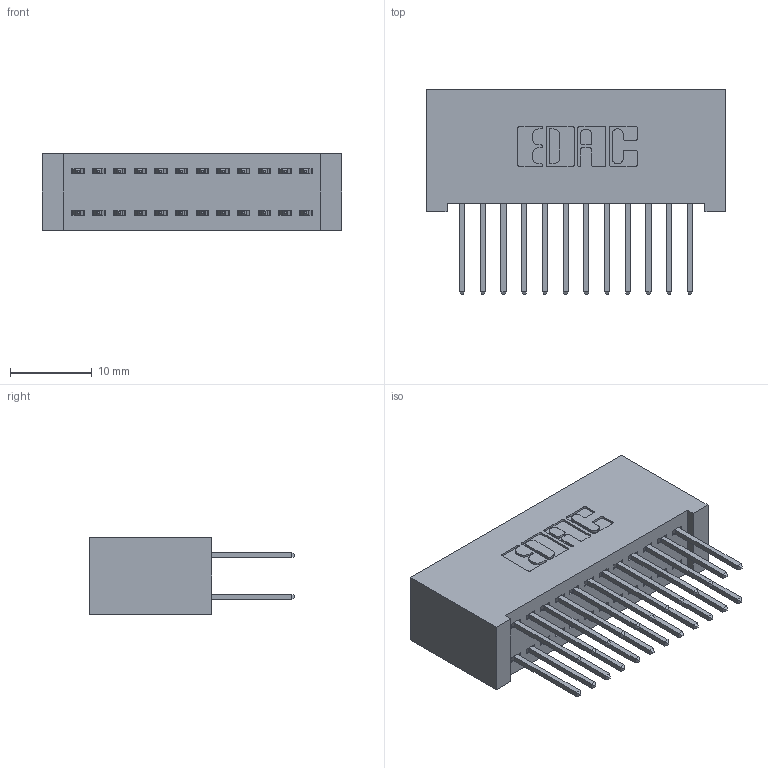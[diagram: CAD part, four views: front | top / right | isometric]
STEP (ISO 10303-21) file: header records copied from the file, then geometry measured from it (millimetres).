
FILE_DESCRIPTION (( 'STEP AP203' ), '1' );
FILE_NAME ('342-024-523-201.STEP', '2018-08-11T02:12:16', ( '' ), ( '' ), 'SwSTEP 2.0', 'SolidWorks 2016', '' );
FILE_SCHEMA (( 'CONFIG_CONTROL_DESIGN' ));
Length unit declared in the file: inch
Products named in the file (3): 342 Part_Lugless; 345-292-001_345-293-123; 342-024-523-201
Assembly tree (25 placements, depth 2):
  342-024-523-201
    342 Part_Lugless
    345-292-001_345-293-123  x24
Bounding box: 36.73 x 25.15 x 9.4 mm (x, y, z)
Volume: 3646.7 mm3; surface area: 5852.3 mm2
Topology: 25 solids, 25 shells, 1350 faces, 3995 edges, 2630 vertices
Faces by surface type: plane 926, cylinder 424
Entity records: 11209 total; most frequent: CARTESIAN_POINT 1890, ORIENTED_EDGE 1826, DIRECTION 1661, EDGE_CURVE 913, LINE 793, VECTOR 793, VERTEX_POINT 606, AXIS2_PLACEMENT_3D 434
